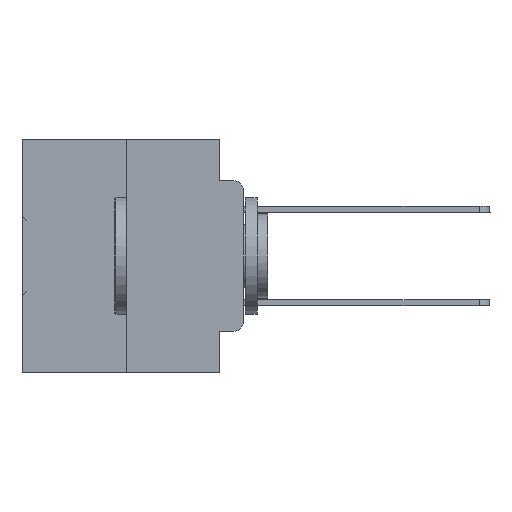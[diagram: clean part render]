
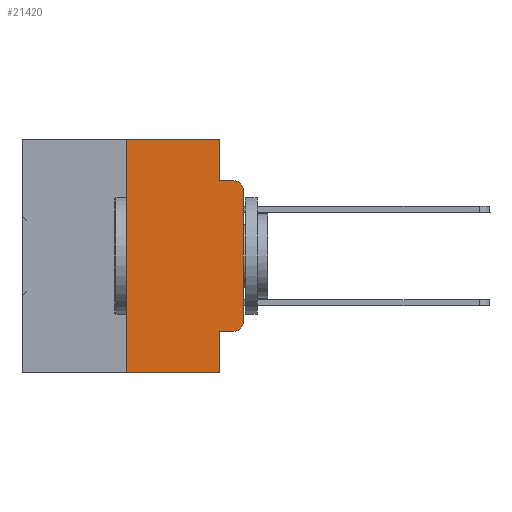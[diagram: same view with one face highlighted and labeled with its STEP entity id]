
A CAD part, left-side view. The second image highlights one B-rep face of the part: STEP entity #21420.
In plain terms, the highlighted planar face has unit normal (-1, 0, 0).
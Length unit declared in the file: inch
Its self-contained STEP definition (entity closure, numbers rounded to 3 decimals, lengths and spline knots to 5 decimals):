
#201 = CARTESIAN_POINT ( 'NONE',  ( 0., 0.051, -0.4115 ) ) ;
#993 = CARTESIAN_POINT ( 'NONE',  ( 0., 0.051, 0. ) ) ;
#1117 = VECTOR ( 'NONE', #11762, 39.37008 ) ;
#1149 = CARTESIAN_POINT ( 'NONE',  ( 0., 0.02, -0.3915 ) ) ;
#1378 = VERTEX_POINT ( 'NONE', #28328 ) ;
#1685 = DIRECTION ( 'NONE',  ( 0., 0., -1. ) ) ;
#2031 = EDGE_CURVE ( 'NONE', #12921, #1378, #26828, .T. ) ;
#2429 = DIRECTION ( 'NONE',  ( 0., -1., 0. ) ) ;
#3271 = CIRCLE ( 'NONE', #26015, 0.02 ) ;
#3333 = VERTEX_POINT ( 'NONE', #14539 ) ;
#3604 = LINE ( 'NONE', #13648, #37647 ) ;
#3923 = EDGE_CURVE ( 'NONE', #3333, #18224, #3604, .T. ) ;
#5089 = ORIENTED_EDGE ( 'NONE', *, *, #38187, .T. ) ;
#5364 = ORIENTED_EDGE ( 'NONE', *, *, #29311, .T. ) ;
#6303 = ORIENTED_EDGE ( 'NONE', *, *, #27365, .T. ) ;
#6785 = DIRECTION ( 'NONE',  ( 0., 0., -1. ) ) ;
#7508 = EDGE_LOOP ( 'NONE', ( #37622, #6303, #27713, #28730, #31447, #38551, #5364, #13192, #29449, #5089 ) ) ;
#7640 = AXIS2_PLACEMENT_3D ( 'NONE', #11630, #8272, #29468 ) ;
#8272 = DIRECTION ( 'NONE',  ( 1., 0., 0. ) ) ;
#8336 = VERTEX_POINT ( 'NONE', #22557 ) ;
#9421 = LINE ( 'NONE', #18911, #31303 ) ;
#10214 = CARTESIAN_POINT ( 'NONE',  ( 0., 0.02, -0.0885 ) ) ;
#11630 = CARTESIAN_POINT ( 'NONE',  ( 0., 0.473, 0. ) ) ;
#11762 = DIRECTION ( 'NONE',  ( 0., -1., 0. ) ) ;
#12354 = CARTESIAN_POINT ( 'NONE',  ( 0., 0.25, 0. ) ) ;
#12921 = VERTEX_POINT ( 'NONE', #201 ) ;
#13192 = ORIENTED_EDGE ( 'NONE', *, *, #37110, .F. ) ;
#13648 = CARTESIAN_POINT ( 'NONE',  ( 0., 0.051, -0.0885 ) ) ;
#14356 = CARTESIAN_POINT ( 'NONE',  ( 0., 0.25, -0.5 ) ) ;
#14539 = CARTESIAN_POINT ( 'NONE',  ( 0., 0.051, -0.0885 ) ) ;
#14727 = CARTESIAN_POINT ( 'NONE',  ( 0., 0.051, -0.4115 ) ) ;
#14950 = CARTESIAN_POINT ( 'NONE',  ( 0., 0.051, 0. ) ) ;
#15300 = VECTOR ( 'NONE', #6785, 39.37008 ) ;
#15458 = DIRECTION ( 'NONE',  ( 0., 0., -1. ) ) ;
#15827 = EDGE_CURVE ( 'NONE', #36483, #3333, #27543, .T. ) ;
#16101 = EDGE_CURVE ( 'NONE', #22377, #23801, #33221, .T. ) ;
#17575 = PLANE ( 'NONE',  #7640 ) ;
#18224 = VERTEX_POINT ( 'NONE', #10214 ) ;
#18911 = CARTESIAN_POINT ( 'NONE',  ( 0., 0.473, 0. ) ) ;
#19955 = CARTESIAN_POINT ( 'NONE',  ( 0., 0., -0.3915 ) ) ;
#20555 = CARTESIAN_POINT ( 'NONE',  ( 0., 0., -0.1085 ) ) ;
#21420 = ADVANCED_FACE ( 'NONE', ( #32461 ), #17575, .F. ) ;
#21708 = VERTEX_POINT ( 'NONE', #37381 ) ;
#21716 = VECTOR ( 'NONE', #15458, 39.37008 ) ;
#22040 = EDGE_CURVE ( 'NONE', #31269, #21708, #27421, .T. ) ;
#22377 = VERTEX_POINT ( 'NONE', #19955 ) ;
#22557 = CARTESIAN_POINT ( 'NONE',  ( 0., 0.051, -0.5 ) ) ;
#22918 = DIRECTION ( 'NONE',  ( -1., 0., 0. ) ) ;
#23713 = CIRCLE ( 'NONE', #31329, 0.02 ) ;
#23801 = VERTEX_POINT ( 'NONE', #20555 ) ;
#24252 = DIRECTION ( 'NONE',  ( 0., 0., 1. ) ) ;
#24480 = CARTESIAN_POINT ( 'NONE',  ( 0., 0., 0. ) ) ;
#24627 = LINE ( 'NONE', #30566, #15300 ) ;
#26015 = AXIS2_PLACEMENT_3D ( 'NONE', #1149, #22918, #31849 ) ;
#26316 = VECTOR ( 'NONE', #2429, 39.37008 ) ;
#26587 = LINE ( 'NONE', #29955, #26316 ) ;
#26828 = LINE ( 'NONE', #14727, #1117 ) ;
#27288 = EDGE_CURVE ( 'NONE', #21708, #36483, #9421, .T. ) ;
#27365 = EDGE_CURVE ( 'NONE', #23801, #18224, #23713, .T. ) ;
#27421 = LINE ( 'NONE', #12354, #36800 ) ;
#27543 = LINE ( 'NONE', #993, #21716 ) ;
#27713 = ORIENTED_EDGE ( 'NONE', *, *, #3923, .F. ) ;
#28328 = CARTESIAN_POINT ( 'NONE',  ( 0., 0.02, -0.4115 ) ) ;
#28730 = ORIENTED_EDGE ( 'NONE', *, *, #15827, .F. ) ;
#29311 = EDGE_CURVE ( 'NONE', #31269, #8336, #26587, .T. ) ;
#29449 = ORIENTED_EDGE ( 'NONE', *, *, #2031, .T. ) ;
#29468 = DIRECTION ( 'NONE',  ( 0., 0., -1. ) ) ;
#29955 = CARTESIAN_POINT ( 'NONE',  ( 0., 0.473, -0.5 ) ) ;
#30566 = CARTESIAN_POINT ( 'NONE',  ( 0., 0.051, 0. ) ) ;
#31269 = VERTEX_POINT ( 'NONE', #14356 ) ;
#31303 = VECTOR ( 'NONE', #33812, 39.37008 ) ;
#31329 = AXIS2_PLACEMENT_3D ( 'NONE', #37753, #37563, #1685 ) ;
#31447 = ORIENTED_EDGE ( 'NONE', *, *, #27288, .F. ) ;
#31849 = DIRECTION ( 'NONE',  ( 0., 0., -1. ) ) ;
#32461 = FACE_OUTER_BOUND ( 'NONE', #7508, .T. ) ;
#33221 = LINE ( 'NONE', #24480, #38762 ) ;
#33426 = DIRECTION ( 'NONE',  ( 0., 0., 1. ) ) ;
#33812 = DIRECTION ( 'NONE',  ( 0., -1., 0. ) ) ;
#34693 = DIRECTION ( 'NONE',  ( 0., -1., 0. ) ) ;
#36483 = VERTEX_POINT ( 'NONE', #14950 ) ;
#36800 = VECTOR ( 'NONE', #24252, 39.37008 ) ;
#37110 = EDGE_CURVE ( 'NONE', #12921, #8336, #24627, .T. ) ;
#37381 = CARTESIAN_POINT ( 'NONE',  ( 0., 0.25, 0. ) ) ;
#37563 = DIRECTION ( 'NONE',  ( -1., 0., 0. ) ) ;
#37622 = ORIENTED_EDGE ( 'NONE', *, *, #16101, .T. ) ;
#37647 = VECTOR ( 'NONE', #34693, 39.37008 ) ;
#37753 = CARTESIAN_POINT ( 'NONE',  ( 0., 0.02, -0.1085 ) ) ;
#38187 = EDGE_CURVE ( 'NONE', #1378, #22377, #3271, .T. ) ;
#38551 = ORIENTED_EDGE ( 'NONE', *, *, #22040, .F. ) ;
#38762 = VECTOR ( 'NONE', #33426, 39.37008 ) ;
